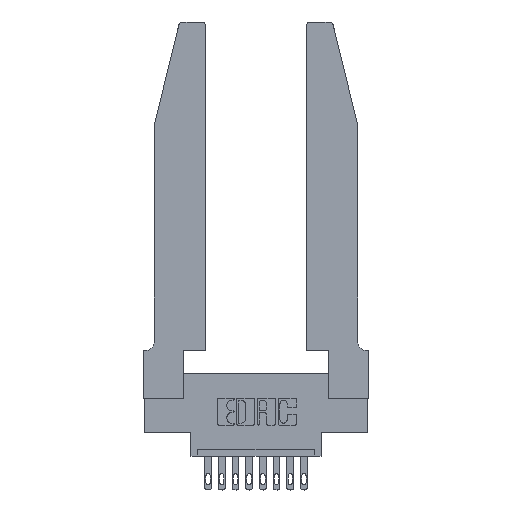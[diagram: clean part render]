
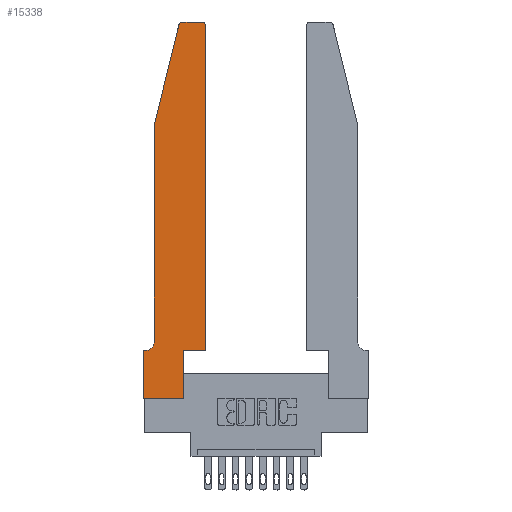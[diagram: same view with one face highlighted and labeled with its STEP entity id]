
A CAD part, top view. The second image highlights one B-rep face of the part: STEP entity #15338.
In plain terms, the highlighted planar face has unit normal (0, 0, 1).
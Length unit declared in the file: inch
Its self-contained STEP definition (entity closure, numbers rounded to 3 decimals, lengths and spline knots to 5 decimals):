
#81 = VECTOR ( 'NONE', #4645, 39.37008 ) ;
#243 = CARTESIAN_POINT ( 'NONE',  ( 0.4205, 2.72, 0.37 ) ) ;
#303 = CARTESIAN_POINT ( 'NONE',  ( 0., 0., 0.37 ) ) ;
#307 = EDGE_CURVE ( 'NONE', #13825, #6811, #12712, .T. ) ;
#552 = CARTESIAN_POINT ( 'NONE',  ( 0.2865, 0., 0.37 ) ) ;
#588 = VECTOR ( 'NONE', #13733, 39.37008 ) ;
#601 = DIRECTION ( 'NONE',  ( 0., -1., 0. ) ) ;
#663 = AXIS2_PLACEMENT_3D ( 'NONE', #3415, #9324, #12894 ) ;
#684 = CARTESIAN_POINT ( 'NONE',  ( 0., 0., 0.37 ) ) ;
#1245 = ORIENTED_EDGE ( 'NONE', *, *, #14889, .T. ) ;
#1304 = FACE_OUTER_BOUND ( 'NONE', #2622, .T. ) ;
#2148 = CARTESIAN_POINT ( 'NONE',  ( 0.2865, 0.35, 0.37 ) ) ;
#2276 = DIRECTION ( 'NONE',  ( -1., 0., 0. ) ) ;
#2481 = ORIENTED_EDGE ( 'NONE', *, *, #13022, .T. ) ;
#2544 = VECTOR ( 'NONE', #6093, 39.37008 ) ;
#2622 = EDGE_LOOP ( 'NONE', ( #7092, #2481, #10606, #10209, #10525, #1245, #7346, #8376, #3784, #11396, #15200, #13585 ) ) ;
#3066 = VECTOR ( 'NONE', #5276, 39.37008 ) ;
#3213 = LINE ( 'NONE', #13273, #9013 ) ;
#3415 = CARTESIAN_POINT ( 'NONE',  ( 0., 0.35, 0.37 ) ) ;
#3425 = EDGE_CURVE ( 'NONE', #3649, #3433, #13947, .T. ) ;
#3433 = VERTEX_POINT ( 'NONE', #552 ) ;
#3557 = DIRECTION ( 'NONE',  ( -0.239, -0.971, 0. ) ) ;
#3649 = VERTEX_POINT ( 'NONE', #684 ) ;
#3784 = ORIENTED_EDGE ( 'NONE', *, *, #9537, .T. ) ;
#4408 = EDGE_CURVE ( 'NONE', #9366, #14290, #6236, .T. ) ;
#4558 = CARTESIAN_POINT ( 'NONE',  ( 0.0055, 0.42, 0.37 ) ) ;
#4645 = DIRECTION ( 'NONE',  ( 1., 0., 0. ) ) ;
#4744 = VECTOR ( 'NONE', #601, 39.37008 ) ;
#4825 = DIRECTION ( 'NONE',  ( 1., 0., 0. ) ) ;
#4916 = CARTESIAN_POINT ( 'NONE',  ( 0.4205, 2.75, 0.37 ) ) ;
#5059 = LINE ( 'NONE', #6593, #588 ) ;
#5276 = DIRECTION ( 'NONE',  ( 0., 1., 0. ) ) ;
#5284 = CARTESIAN_POINT ( 'NONE',  ( 0.4505, 0.35, 0.37 ) ) ;
#5327 = EDGE_CURVE ( 'NONE', #6811, #7614, #3213, .T. ) ;
#5331 = DIRECTION ( 'NONE',  ( 1., 0., 0. ) ) ;
#5344 = EDGE_CURVE ( 'NONE', #11247, #10174, #13333, .T. ) ;
#5653 = CARTESIAN_POINT ( 'NONE',  ( 0.0755, 2., 0.37 ) ) ;
#5788 = CARTESIAN_POINT ( 'NONE',  ( 0.284, 2.75, 0.37 ) ) ;
#6093 = DIRECTION ( 'NONE',  ( 0., -1., 0. ) ) ;
#6236 = LINE ( 'NONE', #8984, #4744 ) ;
#6538 = AXIS2_PLACEMENT_3D ( 'NONE', #4558, #10736, #2276 ) ;
#6593 = CARTESIAN_POINT ( 'NONE',  ( 0.4505, 0.35, 0.37 ) ) ;
#6801 = CARTESIAN_POINT ( 'NONE',  ( 0.284, 2.72, 0.37 ) ) ;
#6811 = VERTEX_POINT ( 'NONE', #4916 ) ;
#7057 = DIRECTION ( 'NONE',  ( 0., 0., 1. ) ) ;
#7092 = ORIENTED_EDGE ( 'NONE', *, *, #5327, .T. ) ;
#7346 = ORIENTED_EDGE ( 'NONE', *, *, #8333, .T. ) ;
#7484 = CARTESIAN_POINT ( 'NONE',  ( 0.4505, 2.72, 0.37 ) ) ;
#7614 = VERTEX_POINT ( 'NONE', #5788 ) ;
#8324 = VERTEX_POINT ( 'NONE', #12065 ) ;
#8326 = CARTESIAN_POINT ( 'NONE',  ( 0.0755, 0.42, 0.37 ) ) ;
#8333 = EDGE_CURVE ( 'NONE', #8503, #3649, #10967, .T. ) ;
#8376 = ORIENTED_EDGE ( 'NONE', *, *, #3425, .T. ) ;
#8503 = VERTEX_POINT ( 'NONE', #13972 ) ;
#8779 = LINE ( 'NONE', #5653, #10115 ) ;
#8793 = VECTOR ( 'NONE', #14608, 39.37008 ) ;
#8984 = CARTESIAN_POINT ( 'NONE',  ( 0.0755, 2., 0.37 ) ) ;
#9013 = VECTOR ( 'NONE', #11918, 39.37008 ) ;
#9178 = LINE ( 'NONE', #10779, #8793 ) ;
#9324 = DIRECTION ( 'NONE',  ( 0., 0., 1. ) ) ;
#9366 = VERTEX_POINT ( 'NONE', #11230 ) ;
#9449 = VECTOR ( 'NONE', #5331, 39.37008 ) ;
#9537 = EDGE_CURVE ( 'NONE', #3433, #11247, #12609, .T. ) ;
#9856 = AXIS2_PLACEMENT_3D ( 'NONE', #243, #12088, #13339 ) ;
#10115 = VECTOR ( 'NONE', #3557, 39.37008 ) ;
#10174 = VERTEX_POINT ( 'NONE', #5284 ) ;
#10209 = ORIENTED_EDGE ( 'NONE', *, *, #4408, .T. ) ;
#10525 = ORIENTED_EDGE ( 'NONE', *, *, #14527, .T. ) ;
#10588 = PLANE ( 'NONE',  #663 ) ;
#10606 = ORIENTED_EDGE ( 'NONE', *, *, #14994, .T. ) ;
#10736 = DIRECTION ( 'NONE',  ( 0., 0., -1. ) ) ;
#10779 = CARTESIAN_POINT ( 'NONE',  ( 0.0755, 0.35, 0.37 ) ) ;
#10869 = CARTESIAN_POINT ( 'NONE',  ( 0., 0., 0.37 ) ) ;
#10967 = LINE ( 'NONE', #10869, #2544 ) ;
#11230 = CARTESIAN_POINT ( 'NONE',  ( 0.0755, 2., 0.37 ) ) ;
#11247 = VERTEX_POINT ( 'NONE', #2148 ) ;
#11256 = CIRCLE ( 'NONE', #6538, 0.07 ) ;
#11338 = AXIS2_PLACEMENT_3D ( 'NONE', #6801, #7057, #4825 ) ;
#11396 = ORIENTED_EDGE ( 'NONE', *, *, #5344, .T. ) ;
#11540 = EDGE_CURVE ( 'NONE', #10174, #13825, #5059, .T. ) ;
#11918 = DIRECTION ( 'NONE',  ( -1., 0., 0. ) ) ;
#11974 = CARTESIAN_POINT ( 'NONE',  ( 0.4505, 0.35, 0.37 ) ) ;
#12065 = CARTESIAN_POINT ( 'NONE',  ( 0.25487, 2.72718, 0.37 ) ) ;
#12088 = DIRECTION ( 'NONE',  ( 0., 0., 1. ) ) ;
#12194 = CARTESIAN_POINT ( 'NONE',  ( 0.2865, 0.35, 0.37 ) ) ;
#12609 = LINE ( 'NONE', #12194, #3066 ) ;
#12712 = CIRCLE ( 'NONE', #9856, 0.03 ) ;
#12894 = DIRECTION ( 'NONE',  ( 1., 0., 0. ) ) ;
#13022 = EDGE_CURVE ( 'NONE', #7614, #8324, #14357, .T. ) ;
#13273 = CARTESIAN_POINT ( 'NONE',  ( 0.2605, 2.75, 0.37 ) ) ;
#13333 = LINE ( 'NONE', #11974, #81 ) ;
#13339 = DIRECTION ( 'NONE',  ( 1., 0., 0. ) ) ;
#13585 = ORIENTED_EDGE ( 'NONE', *, *, #307, .T. ) ;
#13733 = DIRECTION ( 'NONE',  ( 0., 1., 0. ) ) ;
#13825 = VERTEX_POINT ( 'NONE', #7484 ) ;
#13947 = LINE ( 'NONE', #303, #9449 ) ;
#13972 = CARTESIAN_POINT ( 'NONE',  ( 0., 0.35, 0.37 ) ) ;
#14290 = VERTEX_POINT ( 'NONE', #8326 ) ;
#14357 = CIRCLE ( 'NONE', #11338, 0.03 ) ;
#14527 = EDGE_CURVE ( 'NONE', #14290, #14821, #11256, .T. ) ;
#14608 = DIRECTION ( 'NONE',  ( -1., 0., 0. ) ) ;
#14821 = VERTEX_POINT ( 'NONE', #14971 ) ;
#14889 = EDGE_CURVE ( 'NONE', #14821, #8503, #9178, .T. ) ;
#14971 = CARTESIAN_POINT ( 'NONE',  ( 0.0055, 0.35, 0.37 ) ) ;
#14994 = EDGE_CURVE ( 'NONE', #8324, #9366, #8779, .T. ) ;
#15200 = ORIENTED_EDGE ( 'NONE', *, *, #11540, .T. ) ;
#15338 = ADVANCED_FACE ( 'NONE', ( #1304 ), #10588, .T. ) ;
